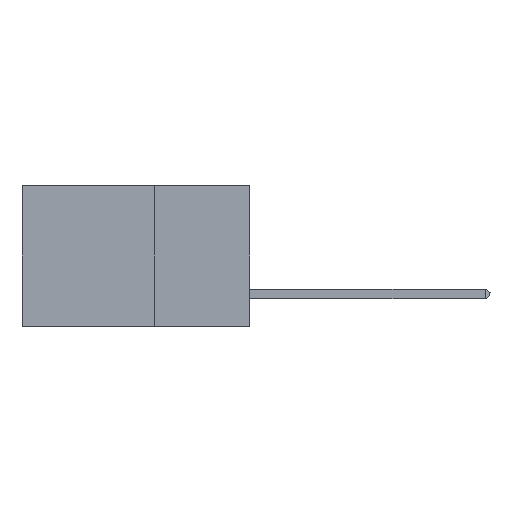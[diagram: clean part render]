
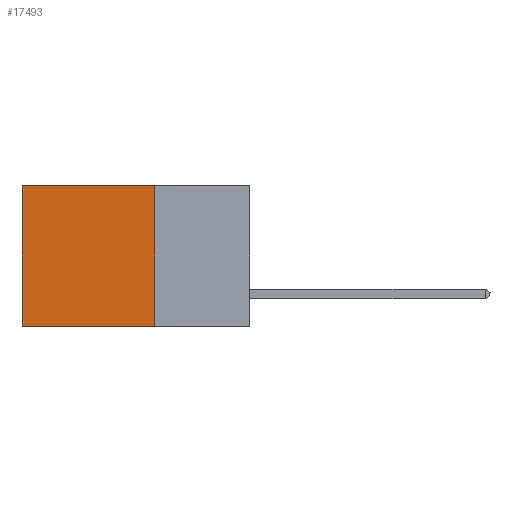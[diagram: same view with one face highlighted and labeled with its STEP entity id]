
A CAD part, left-side view. The second image highlights one B-rep face of the part: STEP entity #17493.
In plain terms, the highlighted planar face has unit normal (-1, 0, 0).
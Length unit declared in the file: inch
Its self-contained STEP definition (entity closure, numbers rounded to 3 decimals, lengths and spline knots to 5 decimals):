
#256 = PLANE ( 'NONE',  #18794 ) ;
#857 = LINE ( 'NONE', #21420, #10353 ) ;
#1166 = DIRECTION ( 'NONE',  ( 0., 0., -1. ) ) ;
#2427 = EDGE_CURVE ( 'NONE', #17685, #19450, #25331, .T. ) ;
#3034 = EDGE_LOOP ( 'NONE', ( #4347, #16866, #10161, #16800 ) ) ;
#4151 = VECTOR ( 'NONE', #5166, 39.37008 ) ;
#4347 = ORIENTED_EDGE ( 'NONE', *, *, #7340, .T. ) ;
#5166 = DIRECTION ( 'NONE',  ( 0., 1., 0. ) ) ;
#5257 = DIRECTION ( 'NONE',  ( 0., 1., 0. ) ) ;
#6100 = CARTESIAN_POINT ( 'NONE',  ( 0.2875, 0.25, 0. ) ) ;
#6820 = LINE ( 'NONE', #6100, #18208 ) ;
#7059 = EDGE_CURVE ( 'NONE', #18029, #21188, #12212, .T. ) ;
#7340 = EDGE_CURVE ( 'NONE', #21188, #19450, #857, .T. ) ;
#7928 = CARTESIAN_POINT ( 'NONE',  ( 0.2875, 0.6, 0. ) ) ;
#9296 = CARTESIAN_POINT ( 'NONE',  ( 0.2875, 0.6, -0.37 ) ) ;
#10161 = ORIENTED_EDGE ( 'NONE', *, *, #11058, .F. ) ;
#10353 = VECTOR ( 'NONE', #14840, 39.37008 ) ;
#11058 = EDGE_CURVE ( 'NONE', #18029, #17685, #6820, .T. ) ;
#11839 = CARTESIAN_POINT ( 'NONE',  ( 0.2875, 0.25, -0.37 ) ) ;
#12212 = LINE ( 'NONE', #28830, #24297 ) ;
#14840 = DIRECTION ( 'NONE',  ( 0., 0., -1. ) ) ;
#16800 = ORIENTED_EDGE ( 'NONE', *, *, #7059, .T. ) ;
#16866 = ORIENTED_EDGE ( 'NONE', *, *, #2427, .F. ) ;
#17493 = ADVANCED_FACE ( 'NONE', ( #27627 ), #256, .F. ) ;
#17685 = VERTEX_POINT ( 'NONE', #21270 ) ;
#18029 = VERTEX_POINT ( 'NONE', #23737 ) ;
#18208 = VECTOR ( 'NONE', #1166, 39.37008 ) ;
#18794 = AXIS2_PLACEMENT_3D ( 'NONE', #26307, #26095, #26416 ) ;
#19450 = VERTEX_POINT ( 'NONE', #9296 ) ;
#21188 = VERTEX_POINT ( 'NONE', #7928 ) ;
#21270 = CARTESIAN_POINT ( 'NONE',  ( 0.2875, 0.25, -0.37 ) ) ;
#21420 = CARTESIAN_POINT ( 'NONE',  ( 0.2875, 0.6, 0. ) ) ;
#23737 = CARTESIAN_POINT ( 'NONE',  ( 0.2875, 0.25, 0. ) ) ;
#24297 = VECTOR ( 'NONE', #5257, 39.37008 ) ;
#25331 = LINE ( 'NONE', #11839, #4151 ) ;
#26095 = DIRECTION ( 'NONE',  ( 1., 0., 0. ) ) ;
#26307 = CARTESIAN_POINT ( 'NONE',  ( 0.2875, 0.25, 0. ) ) ;
#26416 = DIRECTION ( 'NONE',  ( 0., 0., -1. ) ) ;
#27627 = FACE_OUTER_BOUND ( 'NONE', #3034, .T. ) ;
#28830 = CARTESIAN_POINT ( 'NONE',  ( 0.2875, 0.25, 0. ) ) ;
